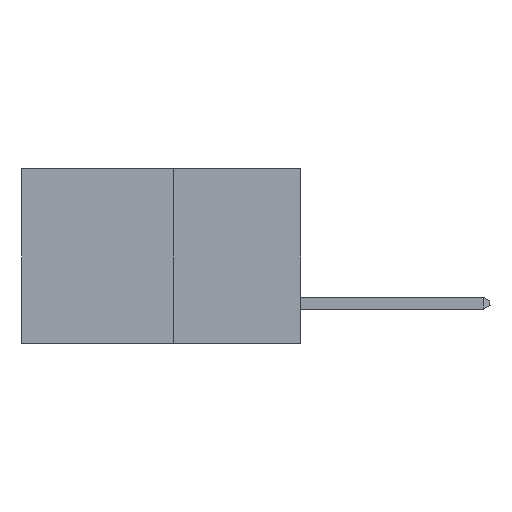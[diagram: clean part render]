
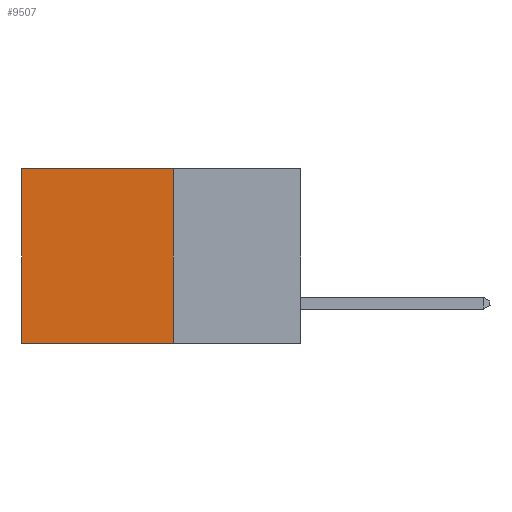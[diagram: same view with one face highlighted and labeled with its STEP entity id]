
A CAD part, left-side view. The second image highlights one B-rep face of the part: STEP entity #9507.
In plain terms, the highlighted planar face has unit normal (-1, 0, 0).
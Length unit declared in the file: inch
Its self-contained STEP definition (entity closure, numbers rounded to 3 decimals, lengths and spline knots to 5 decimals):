
#706 = VERTEX_POINT ( 'NONE', #3363 ) ;
#1030 = FACE_OUTER_BOUND ( 'NONE', #9391, .T. ) ;
#1116 = DIRECTION ( 'NONE',  ( 0., 0., -1. ) ) ;
#1501 = ORIENTED_EDGE ( 'NONE', *, *, #3679, .F. ) ;
#2032 = LINE ( 'NONE', #13124, #8054 ) ;
#2370 = ORIENTED_EDGE ( 'NONE', *, *, #11512, .T. ) ;
#2610 = VECTOR ( 'NONE', #12543, 39.37008 ) ;
#3017 = LINE ( 'NONE', #9042, #2610 ) ;
#3194 = VECTOR ( 'NONE', #10561, 39.37008 ) ;
#3336 = VERTEX_POINT ( 'NONE', #10502 ) ;
#3363 = CARTESIAN_POINT ( 'NONE',  ( 0.277, 0.59, -0.37 ) ) ;
#3587 = LINE ( 'NONE', #13678, #3194 ) ;
#3679 = EDGE_CURVE ( 'NONE', #3336, #5346, #3587, .T. ) ;
#3745 = DIRECTION ( 'NONE',  ( 0., 0., -1. ) ) ;
#4891 = PLANE ( 'NONE',  #7232 ) ;
#4959 = CARTESIAN_POINT ( 'NONE',  ( 0.277, 0.59, -0.37 ) ) ;
#5346 = VERTEX_POINT ( 'NONE', #5988 ) ;
#5988 = CARTESIAN_POINT ( 'NONE',  ( 0.277, 0.27, -0.37 ) ) ;
#6975 = LINE ( 'NONE', #4959, #13598 ) ;
#7232 = AXIS2_PLACEMENT_3D ( 'NONE', #15327, #8393, #1116 ) ;
#7256 = ORIENTED_EDGE ( 'NONE', *, *, #13171, .F. ) ;
#8054 = VECTOR ( 'NONE', #9654, 39.37008 ) ;
#8393 = DIRECTION ( 'NONE',  ( 1., 0., 0. ) ) ;
#8701 = VERTEX_POINT ( 'NONE', #9304 ) ;
#8912 = EDGE_CURVE ( 'NONE', #8701, #706, #6975, .T. ) ;
#9041 = ORIENTED_EDGE ( 'NONE', *, *, #8912, .T. ) ;
#9042 = CARTESIAN_POINT ( 'NONE',  ( 0.277, 0.27, -0.37 ) ) ;
#9304 = CARTESIAN_POINT ( 'NONE',  ( 0.277, 0.59, 0. ) ) ;
#9391 = EDGE_LOOP ( 'NONE', ( #9041, #7256, #1501, #2370 ) ) ;
#9507 = ADVANCED_FACE ( 'NONE', ( #1030 ), #4891, .F. ) ;
#9654 = DIRECTION ( 'NONE',  ( 0., 1., 0. ) ) ;
#10502 = CARTESIAN_POINT ( 'NONE',  ( 0.277, 0.27, 0. ) ) ;
#10561 = DIRECTION ( 'NONE',  ( 0., 0., -1. ) ) ;
#11512 = EDGE_CURVE ( 'NONE', #3336, #8701, #2032, .T. ) ;
#12543 = DIRECTION ( 'NONE',  ( 0., 1., 0. ) ) ;
#13124 = CARTESIAN_POINT ( 'NONE',  ( 0.277, 0.27, 0. ) ) ;
#13171 = EDGE_CURVE ( 'NONE', #5346, #706, #3017, .T. ) ;
#13598 = VECTOR ( 'NONE', #3745, 39.37008 ) ;
#13678 = CARTESIAN_POINT ( 'NONE',  ( 0.277, 0.27, -0.37 ) ) ;
#15327 = CARTESIAN_POINT ( 'NONE',  ( 0.277, 0.27, -0.37 ) ) ;
